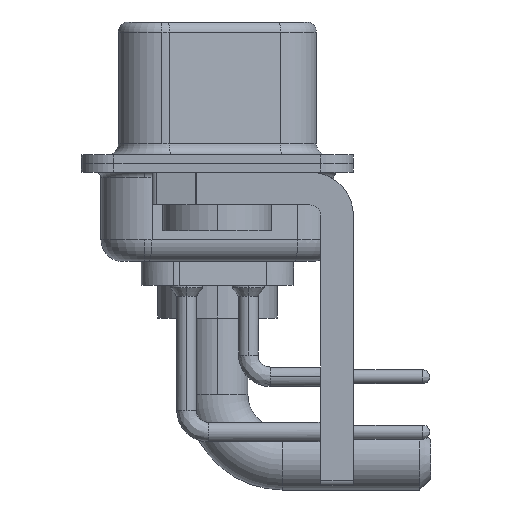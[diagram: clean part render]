
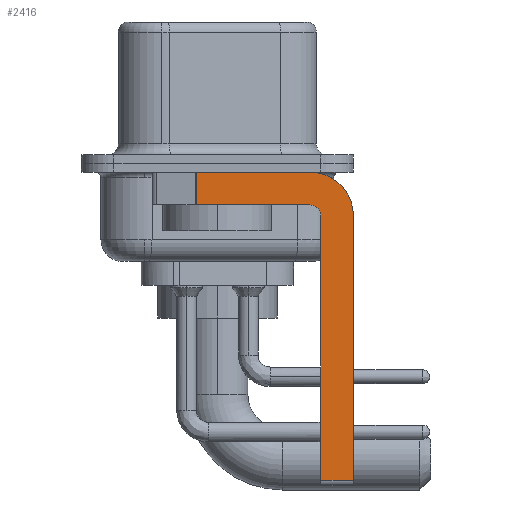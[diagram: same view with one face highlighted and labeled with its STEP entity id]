
A CAD part, left-side view. The second image highlights one B-rep face of the part: STEP entity #2416.
In plain terms, the highlighted planar face has unit normal (-1, 0, 0).
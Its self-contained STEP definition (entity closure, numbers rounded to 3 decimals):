
#988 = CARTESIAN_POINT ( 'NONE',  ( -2.9, -4.25, -1.9 ) ) ;
#1172 = AXIS2_PLACEMENT_3D ( 'NONE', #8594, #15776, #16131 ) ;
#1245 = LINE ( 'NONE', #8461, #11029 ) ;
#1574 = EDGE_CURVE ( 'NONE', #7373, #18095, #11369, .T. ) ;
#1647 = CARTESIAN_POINT ( 'NONE',  ( -2.9, -4.25, -0.4 ) ) ;
#1758 = DIRECTION ( 'NONE',  ( 0., 0., -1. ) ) ;
#1832 = CARTESIAN_POINT ( 'NONE',  ( -2.9, 0.978, -1.9 ) ) ;
#1916 = EDGE_LOOP ( 'NONE', ( #6077, #7232, #22401, #19164, #13942, #4113, #7807, #2908 ) ) ;
#2175 = CARTESIAN_POINT ( 'NONE',  ( -2.9, -4.25, -1.9 ) ) ;
#2416 = ADVANCED_FACE ( 'NONE', ( #15940 ), #22990, .F. ) ;
#2859 = CARTESIAN_POINT ( 'NONE',  ( -2.9, 0.978, -0.4 ) ) ;
#2908 = ORIENTED_EDGE ( 'NONE', *, *, #1574, .F. ) ;
#3305 = DIRECTION ( 'NONE',  ( 1., 0., 0. ) ) ;
#3755 = CARTESIAN_POINT ( 'NONE',  ( -2.9, -4.25, -2.4 ) ) ;
#4113 = ORIENTED_EDGE ( 'NONE', *, *, #14461, .T. ) ;
#4307 = VECTOR ( 'NONE', #10518, 1000. ) ;
#6077 = ORIENTED_EDGE ( 'NONE', *, *, #22596, .F. ) ;
#6118 = VECTOR ( 'NONE', #13622, 1000. ) ;
#6279 = CARTESIAN_POINT ( 'NONE',  ( -2.9, -4.75, -14.55 ) ) ;
#6568 = DIRECTION ( 'NONE',  ( 0., 0., -1. ) ) ;
#6659 = DIRECTION ( 'NONE',  ( 0., 0., 1. ) ) ;
#7080 = LINE ( 'NONE', #21253, #4307 ) ;
#7232 = ORIENTED_EDGE ( 'NONE', *, *, #18452, .T. ) ;
#7323 = EDGE_CURVE ( 'NONE', #18095, #18536, #22870, .T. ) ;
#7373 = VERTEX_POINT ( 'NONE', #1647 ) ;
#7586 = VERTEX_POINT ( 'NONE', #9774 ) ;
#7807 = ORIENTED_EDGE ( 'NONE', *, *, #7323, .F. ) ;
#7873 = LINE ( 'NONE', #16839, #19567 ) ;
#8359 = CIRCLE ( 'NONE', #16998, 0.5 ) ;
#8461 = CARTESIAN_POINT ( 'NONE',  ( -2.9, -4.75, -14.8 ) ) ;
#8594 = CARTESIAN_POINT ( 'NONE',  ( -2.9, -4.25, -2.4 ) ) ;
#8969 = DIRECTION ( 'NONE',  ( -1., 0., 0. ) ) ;
#9774 = CARTESIAN_POINT ( 'NONE',  ( -2.9, -4.75, -2.4 ) ) ;
#10394 = DIRECTION ( 'NONE',  ( 0., 0., -1. ) ) ;
#10518 = DIRECTION ( 'NONE',  ( 0., -1., 0. ) ) ;
#11029 = VECTOR ( 'NONE', #6659, 1000. ) ;
#11278 = DIRECTION ( 'NONE',  ( 0., -1., 0. ) ) ;
#11369 = CIRCLE ( 'NONE', #1172, 2. ) ;
#11938 = AXIS2_PLACEMENT_3D ( 'NONE', #19349, #3305, #1758 ) ;
#12655 = EDGE_CURVE ( 'NONE', #17355, #22621, #15166, .T. ) ;
#12845 = DIRECTION ( 'NONE',  ( 0., 0., 1. ) ) ;
#12990 = VECTOR ( 'NONE', #11278, 1000. ) ;
#13321 = CARTESIAN_POINT ( 'NONE',  ( -2.9, -6.25, -14.55 ) ) ;
#13622 = DIRECTION ( 'NONE',  ( 0., 1., 0. ) ) ;
#13942 = ORIENTED_EDGE ( 'NONE', *, *, #15917, .F. ) ;
#14309 = VERTEX_POINT ( 'NONE', #2859 ) ;
#14461 = EDGE_CURVE ( 'NONE', #19427, #18536, #7080, .T. ) ;
#15026 = EDGE_CURVE ( 'NONE', #7586, #17355, #8359, .T. ) ;
#15166 = LINE ( 'NONE', #988, #6118 ) ;
#15776 = DIRECTION ( 'NONE',  ( 1., 0., 0. ) ) ;
#15917 = EDGE_CURVE ( 'NONE', #19427, #7586, #1245, .T. ) ;
#15940 = FACE_OUTER_BOUND ( 'NONE', #1916, .T. ) ;
#16131 = DIRECTION ( 'NONE',  ( 0., 0., -1. ) ) ;
#16839 = CARTESIAN_POINT ( 'NONE',  ( -2.9, 0.978, -1.9 ) ) ;
#16998 = AXIS2_PLACEMENT_3D ( 'NONE', #3755, #8969, #12845 ) ;
#17355 = VERTEX_POINT ( 'NONE', #2175 ) ;
#17684 = VECTOR ( 'NONE', #10394, 1000. ) ;
#17997 = CARTESIAN_POINT ( 'NONE',  ( -2.9, 3., -0.4 ) ) ;
#18095 = VERTEX_POINT ( 'NONE', #22866 ) ;
#18452 = EDGE_CURVE ( 'NONE', #14309, #22621, #7873, .T. ) ;
#18536 = VERTEX_POINT ( 'NONE', #13321 ) ;
#19164 = ORIENTED_EDGE ( 'NONE', *, *, #15026, .F. ) ;
#19349 = CARTESIAN_POINT ( 'NONE',  ( -2.9, -4.25, -2.4 ) ) ;
#19427 = VERTEX_POINT ( 'NONE', #6279 ) ;
#19567 = VECTOR ( 'NONE', #6568, 1000. ) ;
#19880 = LINE ( 'NONE', #17997, #12990 ) ;
#21227 = CARTESIAN_POINT ( 'NONE',  ( -2.9, -6.25, -2.4 ) ) ;
#21253 = CARTESIAN_POINT ( 'NONE',  ( -2.9, -4.25, -14.55 ) ) ;
#22401 = ORIENTED_EDGE ( 'NONE', *, *, #12655, .F. ) ;
#22596 = EDGE_CURVE ( 'NONE', #14309, #7373, #19880, .T. ) ;
#22621 = VERTEX_POINT ( 'NONE', #1832 ) ;
#22866 = CARTESIAN_POINT ( 'NONE',  ( -2.9, -6.25, -2.4 ) ) ;
#22870 = LINE ( 'NONE', #21227, #17684 ) ;
#22990 = PLANE ( 'NONE',  #11938 ) ;
